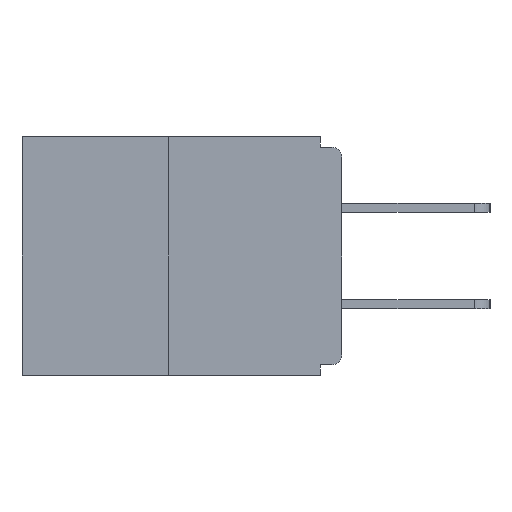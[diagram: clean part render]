
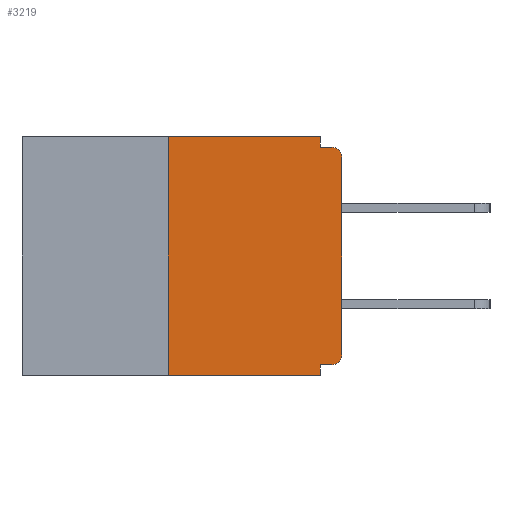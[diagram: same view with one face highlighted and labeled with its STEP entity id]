
A CAD part, left-side view. The second image highlights one B-rep face of the part: STEP entity #3219.
In plain terms, the highlighted planar face has unit normal (-1, 0, 0).
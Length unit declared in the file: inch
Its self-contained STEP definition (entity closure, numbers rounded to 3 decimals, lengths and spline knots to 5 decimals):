
#23 = EDGE_CURVE ( 'NONE', #4748, #7295, #17658, .T. ) ;
#205 = AXIS2_PLACEMENT_3D ( 'NONE', #1191, #11600, #7117 ) ;
#1124 = VERTEX_POINT ( 'NONE', #5370 ) ;
#1191 = CARTESIAN_POINT ( 'NONE',  ( 0., 0.015, -0.313 ) ) ;
#1267 = PLANE ( 'NONE',  #17277 ) ;
#1417 = CARTESIAN_POINT ( 'NONE',  ( 0., 0.031, -0.015 ) ) ;
#1428 = CARTESIAN_POINT ( 'NONE',  ( 0., 0., -0.015 ) ) ;
#1469 = CARTESIAN_POINT ( 'NONE',  ( 0., 0.46, 0. ) ) ;
#1521 = LINE ( 'NONE', #1428, #12683 ) ;
#2038 = DIRECTION ( 'NONE',  ( 0., 1., 0. ) ) ;
#3021 = ORIENTED_EDGE ( 'NONE', *, *, #10651, .F. ) ;
#3219 = ADVANCED_FACE ( 'NONE', ( #18656 ), #1267, .F. ) ;
#3397 = ORIENTED_EDGE ( 'NONE', *, *, #7837, .T. ) ;
#3503 = VECTOR ( 'NONE', #2038, 39.37008 ) ;
#3749 = LINE ( 'NONE', #7773, #3503 ) ;
#3866 = ORIENTED_EDGE ( 'NONE', *, *, #6460, .F. ) ;
#4214 = CARTESIAN_POINT ( 'NONE',  ( 0., 0., 0. ) ) ;
#4321 = CARTESIAN_POINT ( 'NONE',  ( 0., 0.031, 0. ) ) ;
#4748 = VERTEX_POINT ( 'NONE', #15544 ) ;
#5012 = DIRECTION ( 'NONE',  ( 0., 0., -1. ) ) ;
#5097 = EDGE_CURVE ( 'NONE', #14028, #9613, #11210, .T. ) ;
#5169 = CARTESIAN_POINT ( 'NONE',  ( 0., 0.015, -0.015 ) ) ;
#5370 = CARTESIAN_POINT ( 'NONE',  ( 0., 0.031, 0. ) ) ;
#5424 = DIRECTION ( 'NONE',  ( 0., -1., 0. ) ) ;
#5559 = VECTOR ( 'NONE', #11609, 39.37008 ) ;
#5600 = LINE ( 'NONE', #18870, #5559 ) ;
#6164 = DIRECTION ( 'NONE',  ( -1., 0., 0. ) ) ;
#6372 = EDGE_CURVE ( 'NONE', #9613, #1124, #17203, .T. ) ;
#6408 = AXIS2_PLACEMENT_3D ( 'NONE', #12177, #6164, #5012 ) ;
#6460 = EDGE_CURVE ( 'NONE', #1124, #10046, #17393, .T. ) ;
#7082 = EDGE_CURVE ( 'NONE', #16604, #4748, #7570, .T. ) ;
#7117 = DIRECTION ( 'NONE',  ( 0., 0., -1. ) ) ;
#7295 = VERTEX_POINT ( 'NONE', #5169 ) ;
#7306 = DIRECTION ( 'NONE',  ( 0., 0., -1. ) ) ;
#7441 = VECTOR ( 'NONE', #9850, 39.37008 ) ;
#7460 = DIRECTION ( 'NONE',  ( 0., 0., 1. ) ) ;
#7464 = CARTESIAN_POINT ( 'NONE',  ( 0., 0.25, 0. ) ) ;
#7570 = LINE ( 'NONE', #4214, #17868 ) ;
#7773 = CARTESIAN_POINT ( 'NONE',  ( 0., 0., -0.328 ) ) ;
#7832 = ORIENTED_EDGE ( 'NONE', *, *, #18719, .F. ) ;
#7837 = EDGE_CURVE ( 'NONE', #14028, #8040, #8100, .T. ) ;
#7924 = ORIENTED_EDGE ( 'NONE', *, *, #12376, .F. ) ;
#8040 = VERTEX_POINT ( 'NONE', #13048 ) ;
#8100 = LINE ( 'NONE', #18585, #9696 ) ;
#8797 = EDGE_CURVE ( 'NONE', #12691, #16604, #12129, .T. ) ;
#8931 = VERTEX_POINT ( 'NONE', #12549 ) ;
#9613 = VERTEX_POINT ( 'NONE', #7464 ) ;
#9624 = VECTOR ( 'NONE', #10139, 39.37008 ) ;
#9696 = VECTOR ( 'NONE', #5424, 39.37008 ) ;
#9764 = DIRECTION ( 'NONE',  ( 0., -1., 0. ) ) ;
#9802 = ORIENTED_EDGE ( 'NONE', *, *, #23, .T. ) ;
#9850 = DIRECTION ( 'NONE',  ( 0., 0., 1. ) ) ;
#10046 = VERTEX_POINT ( 'NONE', #1417 ) ;
#10139 = DIRECTION ( 'NONE',  ( 0., 0., -1. ) ) ;
#10353 = DIRECTION ( 'NONE',  ( 1., 0., 0. ) ) ;
#10537 = VECTOR ( 'NONE', #9764, 39.37008 ) ;
#10651 = EDGE_CURVE ( 'NONE', #12691, #8931, #3749, .T. ) ;
#11113 = ORIENTED_EDGE ( 'NONE', *, *, #7082, .T. ) ;
#11210 = LINE ( 'NONE', #17103, #7441 ) ;
#11600 = DIRECTION ( 'NONE',  ( -1., 0., 0. ) ) ;
#11609 = DIRECTION ( 'NONE',  ( 0., 0., -1. ) ) ;
#11706 = CARTESIAN_POINT ( 'NONE',  ( 0., 0., -0.313 ) ) ;
#12129 = CIRCLE ( 'NONE', #205, 0.015 ) ;
#12177 = CARTESIAN_POINT ( 'NONE',  ( 0., 0.015, -0.03 ) ) ;
#12376 = EDGE_CURVE ( 'NONE', #10046, #7295, #1521, .T. ) ;
#12549 = CARTESIAN_POINT ( 'NONE',  ( 0., 0.031, -0.328 ) ) ;
#12683 = VECTOR ( 'NONE', #16040, 39.37008 ) ;
#12691 = VERTEX_POINT ( 'NONE', #15549 ) ;
#13048 = CARTESIAN_POINT ( 'NONE',  ( 0., 0.031, -0.343 ) ) ;
#14028 = VERTEX_POINT ( 'NONE', #18645 ) ;
#14257 = CARTESIAN_POINT ( 'NONE',  ( 0., 0.46, 0. ) ) ;
#15544 = CARTESIAN_POINT ( 'NONE',  ( 0., 0., -0.03 ) ) ;
#15549 = CARTESIAN_POINT ( 'NONE',  ( 0., 0.015, -0.328 ) ) ;
#16040 = DIRECTION ( 'NONE',  ( 0., -1., 0. ) ) ;
#16292 = EDGE_LOOP ( 'NONE', ( #16975, #16316, #3397, #7832, #3021, #16864, #11113, #9802, #7924, #3866 ) ) ;
#16316 = ORIENTED_EDGE ( 'NONE', *, *, #5097, .F. ) ;
#16604 = VERTEX_POINT ( 'NONE', #11706 ) ;
#16864 = ORIENTED_EDGE ( 'NONE', *, *, #8797, .T. ) ;
#16975 = ORIENTED_EDGE ( 'NONE', *, *, #6372, .F. ) ;
#17103 = CARTESIAN_POINT ( 'NONE',  ( 0., 0.25, 0. ) ) ;
#17203 = LINE ( 'NONE', #14257, #10537 ) ;
#17277 = AXIS2_PLACEMENT_3D ( 'NONE', #1469, #10353, #7306 ) ;
#17393 = LINE ( 'NONE', #4321, #9624 ) ;
#17658 = CIRCLE ( 'NONE', #6408, 0.015 ) ;
#17868 = VECTOR ( 'NONE', #7460, 39.37008 ) ;
#18585 = CARTESIAN_POINT ( 'NONE',  ( 0., 0.46, -0.343 ) ) ;
#18645 = CARTESIAN_POINT ( 'NONE',  ( 0., 0.25, -0.343 ) ) ;
#18656 = FACE_OUTER_BOUND ( 'NONE', #16292, .T. ) ;
#18719 = EDGE_CURVE ( 'NONE', #8931, #8040, #5600, .T. ) ;
#18870 = CARTESIAN_POINT ( 'NONE',  ( 0., 0.031, -0.343 ) ) ;
